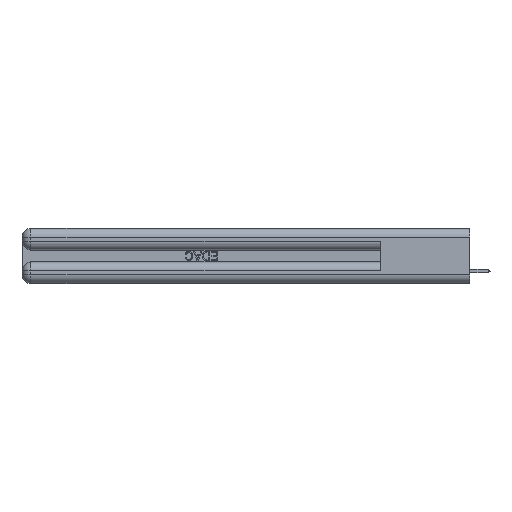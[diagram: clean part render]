
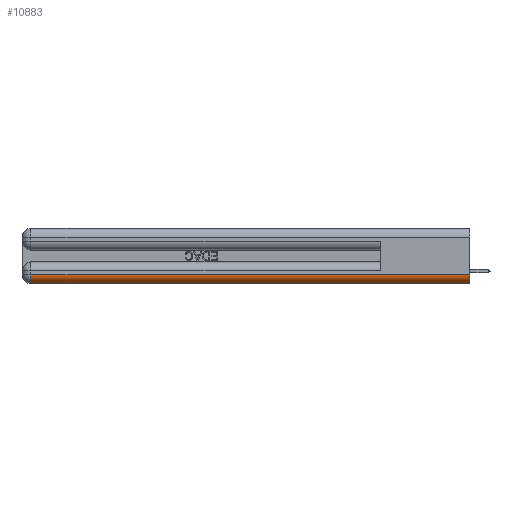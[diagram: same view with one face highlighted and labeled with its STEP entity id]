
A CAD part, left-side view. The second image highlights one B-rep face of the part: STEP entity #10883.
In plain terms, the highlighted cylindrical face has radius 1.524 mm (diameter 3.048 mm), a partial arc.
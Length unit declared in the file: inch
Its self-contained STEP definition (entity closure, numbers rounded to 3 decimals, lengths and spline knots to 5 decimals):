
#1439 = CARTESIAN_POINT ( 'NONE',  ( 0.06, 0., 0. ) ) ;
#4864 = VERTEX_POINT ( 'NONE', #46601 ) ;
#5559 = DIRECTION ( 'NONE',  ( 0., 0., 1. ) ) ;
#5568 = ORIENTED_EDGE ( 'NONE', *, *, #6281, .F. ) ;
#6006 = CIRCLE ( 'NONE', #18244, 0.06 ) ;
#6281 = EDGE_CURVE ( 'NONE', #7313, #27644, #22906, .T. ) ;
#7313 = VERTEX_POINT ( 'NONE', #47868 ) ;
#7611 = EDGE_CURVE ( 'NONE', #41392, #7313, #23260, .T. ) ;
#8619 = CARTESIAN_POINT ( 'NONE',  ( 0., 2.94, 0.06 ) ) ;
#9685 = DIRECTION ( 'NONE',  ( 0., 1., 0. ) ) ;
#10883 = ADVANCED_FACE ( 'NONE', ( #30168 ), #32858, .T. ) ;
#11044 = DIRECTION ( 'NONE',  ( 0., -1., 0. ) ) ;
#11582 = CARTESIAN_POINT ( 'NONE',  ( 0.06, 3., 0. ) ) ;
#16379 = ORIENTED_EDGE ( 'NONE', *, *, #30844, .F. ) ;
#17082 = AXIS2_PLACEMENT_3D ( 'NONE', #29969, #42546, #5559 ) ;
#18244 = AXIS2_PLACEMENT_3D ( 'NONE', #49466, #27940, #49094 ) ;
#19041 = CARTESIAN_POINT ( 'NONE',  ( 0., 0., 0.06 ) ) ;
#22906 = CIRCLE ( 'NONE', #17082, 0.06 ) ;
#23260 = LINE ( 'NONE', #11582, #33920 ) ;
#24184 = LINE ( 'NONE', #19041, #42937 ) ;
#24255 = DIRECTION ( 'NONE',  ( 0., 1., 0. ) ) ;
#27644 = VERTEX_POINT ( 'NONE', #8619 ) ;
#27940 = DIRECTION ( 'NONE',  ( 0., -1., 0. ) ) ;
#29969 = CARTESIAN_POINT ( 'NONE',  ( 0.06, 2.94, 0.06 ) ) ;
#30168 = FACE_OUTER_BOUND ( 'NONE', #52530, .T. ) ;
#30844 = EDGE_CURVE ( 'NONE', #4864, #41392, #6006, .T. ) ;
#32858 = CYLINDRICAL_SURFACE ( 'NONE', #43121, 0.06 ) ;
#33920 = VECTOR ( 'NONE', #24255, 39.37008 ) ;
#41392 = VERTEX_POINT ( 'NONE', #1439 ) ;
#42546 = DIRECTION ( 'NONE',  ( 0., 1., 0. ) ) ;
#42937 = VECTOR ( 'NONE', #11044, 39.37008 ) ;
#43121 = AXIS2_PLACEMENT_3D ( 'NONE', #43692, #9685, #52126 ) ;
#43692 = CARTESIAN_POINT ( 'NONE',  ( 0.06, 0., 0.06 ) ) ;
#46601 = CARTESIAN_POINT ( 'NONE',  ( 0., 0., 0.06 ) ) ;
#47868 = CARTESIAN_POINT ( 'NONE',  ( 0.06, 2.94, 0. ) ) ;
#49094 = DIRECTION ( 'NONE',  ( 0., 0., 1. ) ) ;
#49466 = CARTESIAN_POINT ( 'NONE',  ( 0.06, 0., 0.06 ) ) ;
#50116 = ORIENTED_EDGE ( 'NONE', *, *, #50483, .F. ) ;
#50483 = EDGE_CURVE ( 'NONE', #27644, #4864, #24184, .T. ) ;
#52126 = DIRECTION ( 'NONE',  ( 0., 0., 1. ) ) ;
#52176 = ORIENTED_EDGE ( 'NONE', *, *, #7611, .F. ) ;
#52530 = EDGE_LOOP ( 'NONE', ( #16379, #50116, #5568, #52176 ) ) ;
